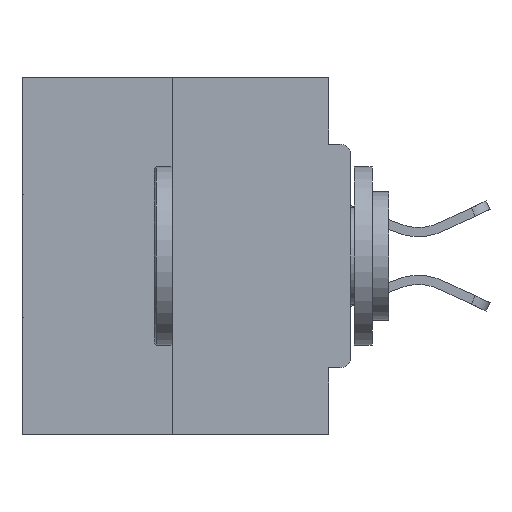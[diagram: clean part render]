
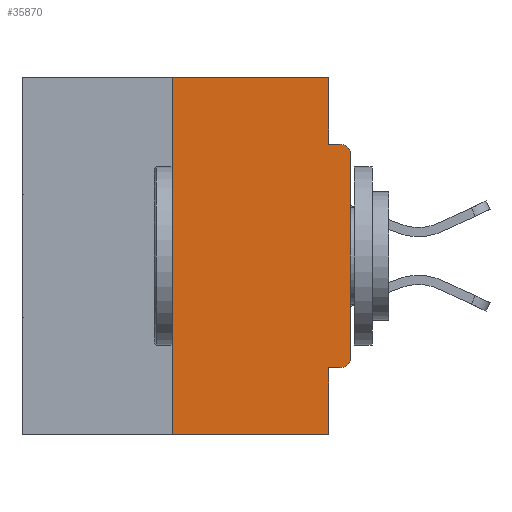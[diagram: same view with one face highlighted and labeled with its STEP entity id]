
A CAD part, left-side view. The second image highlights one B-rep face of the part: STEP entity #35870.
In plain terms, the highlighted planar face has unit normal (-1, 0, 0).
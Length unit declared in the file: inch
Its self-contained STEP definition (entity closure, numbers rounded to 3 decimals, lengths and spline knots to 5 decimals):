
#482 = VECTOR ( 'NONE', #6806, 39.37008 ) ;
#489 = EDGE_CURVE ( 'NONE', #1452, #10768, #7346, .T. ) ;
#610 = CARTESIAN_POINT ( 'NONE',  ( 0., 0.46, 0. ) ) ;
#1418 = CIRCLE ( 'NONE', #18785, 0.015 ) ;
#1452 = VERTEX_POINT ( 'NONE', #18834 ) ;
#1830 = DIRECTION ( 'NONE',  ( 0., -1., 0. ) ) ;
#2419 = CARTESIAN_POINT ( 'NONE',  ( 0., 0.031, 0. ) ) ;
#2492 = DIRECTION ( 'NONE',  ( 0., 0., -1. ) ) ;
#2782 = LINE ( 'NONE', #28223, #5684 ) ;
#2918 = VECTOR ( 'NONE', #22101, 39.37008 ) ;
#3023 = CARTESIAN_POINT ( 'NONE',  ( 0., 0.031, -0.5 ) ) ;
#3658 = EDGE_LOOP ( 'NONE', ( #23017, #25020, #5310, #17488, #17247, #20203, #36136, #10090, #22622, #37999 ) ) ;
#3687 = LINE ( 'NONE', #31050, #36047 ) ;
#4527 = LINE ( 'NONE', #3023, #8351 ) ;
#5092 = CARTESIAN_POINT ( 'NONE',  ( 0., 0.015, -0.3915 ) ) ;
#5310 = ORIENTED_EDGE ( 'NONE', *, *, #18344, .T. ) ;
#5544 = VERTEX_POINT ( 'NONE', #32115 ) ;
#5684 = VECTOR ( 'NONE', #31275, 39.37008 ) ;
#6282 = DIRECTION ( 'NONE',  ( 1., 0., 0. ) ) ;
#6806 = DIRECTION ( 'NONE',  ( 0., 0., 1. ) ) ;
#6832 = DIRECTION ( 'NONE',  ( 0., -1., 0. ) ) ;
#7287 = EDGE_CURVE ( 'NONE', #21469, #35300, #1418, .T. ) ;
#7346 = LINE ( 'NONE', #32718, #31035 ) ;
#7700 = LINE ( 'NONE', #34880, #482 ) ;
#7784 = LINE ( 'NONE', #2419, #22694 ) ;
#8351 = VECTOR ( 'NONE', #2492, 39.37008 ) ;
#9237 = VERTEX_POINT ( 'NONE', #31404 ) ;
#9278 = CARTESIAN_POINT ( 'NONE',  ( 0., 0., -0.4065 ) ) ;
#9405 = FACE_OUTER_BOUND ( 'NONE', #3658, .T. ) ;
#9901 = EDGE_CURVE ( 'NONE', #18406, #30310, #11078, .T. ) ;
#10090 = ORIENTED_EDGE ( 'NONE', *, *, #38746, .T. ) ;
#10210 = LINE ( 'NONE', #9278, #2918 ) ;
#10768 = VERTEX_POINT ( 'NONE', #24532 ) ;
#11078 = LINE ( 'NONE', #610, #33749 ) ;
#11183 = DIRECTION ( 'NONE',  ( 0., 0., -1. ) ) ;
#15640 = DIRECTION ( 'NONE',  ( 0., 0., -1. ) ) ;
#16112 = EDGE_CURVE ( 'NONE', #21469, #9237, #10210, .T. ) ;
#17247 = ORIENTED_EDGE ( 'NONE', *, *, #16112, .F. ) ;
#17488 = ORIENTED_EDGE ( 'NONE', *, *, #20269, .F. ) ;
#18344 = EDGE_CURVE ( 'NONE', #21398, #5544, #2782, .T. ) ;
#18406 = VERTEX_POINT ( 'NONE', #30561 ) ;
#18758 = PLANE ( 'NONE',  #30867 ) ;
#18785 = AXIS2_PLACEMENT_3D ( 'NONE', #5092, #36119, #11183 ) ;
#18821 = EDGE_CURVE ( 'NONE', #21398, #18406, #3687, .T. ) ;
#18834 = CARTESIAN_POINT ( 'NONE',  ( 0., 0.031, -0.0935 ) ) ;
#20203 = ORIENTED_EDGE ( 'NONE', *, *, #7287, .T. ) ;
#20269 = EDGE_CURVE ( 'NONE', #9237, #5544, #4527, .T. ) ;
#20296 = CARTESIAN_POINT ( 'NONE',  ( 0., 0., -0.1085 ) ) ;
#21398 = VERTEX_POINT ( 'NONE', #21840 ) ;
#21469 = VERTEX_POINT ( 'NONE', #26148 ) ;
#21644 = CARTESIAN_POINT ( 'NONE',  ( 0., 0.031, 0. ) ) ;
#21840 = CARTESIAN_POINT ( 'NONE',  ( 0., 0.25, -0.5 ) ) ;
#21857 = EDGE_CURVE ( 'NONE', #30310, #1452, #7784, .T. ) ;
#21949 = DIRECTION ( 'NONE',  ( 0., 0., -1. ) ) ;
#22101 = DIRECTION ( 'NONE',  ( 0., 1., 0. ) ) ;
#22309 = VERTEX_POINT ( 'NONE', #20296 ) ;
#22622 = ORIENTED_EDGE ( 'NONE', *, *, #489, .F. ) ;
#22694 = VECTOR ( 'NONE', #24458, 39.37008 ) ;
#22812 = DIRECTION ( 'NONE',  ( 0., 0., 1. ) ) ;
#23017 = ORIENTED_EDGE ( 'NONE', *, *, #9901, .F. ) ;
#23044 = EDGE_CURVE ( 'NONE', #35300, #22309, #7700, .T. ) ;
#24458 = DIRECTION ( 'NONE',  ( 0., 0., -1. ) ) ;
#24532 = CARTESIAN_POINT ( 'NONE',  ( 0., 0.015, -0.0935 ) ) ;
#24546 = DIRECTION ( 'NONE',  ( -1., 0., 0. ) ) ;
#24798 = CARTESIAN_POINT ( 'NONE',  ( 0., 0.46, 0. ) ) ;
#25020 = ORIENTED_EDGE ( 'NONE', *, *, #18821, .F. ) ;
#26148 = CARTESIAN_POINT ( 'NONE',  ( 0., 0.015, -0.4065 ) ) ;
#27881 = AXIS2_PLACEMENT_3D ( 'NONE', #33362, #24546, #15640 ) ;
#28223 = CARTESIAN_POINT ( 'NONE',  ( 0., 0.46, -0.5 ) ) ;
#30310 = VERTEX_POINT ( 'NONE', #21644 ) ;
#30561 = CARTESIAN_POINT ( 'NONE',  ( 0., 0.25, 0. ) ) ;
#30867 = AXIS2_PLACEMENT_3D ( 'NONE', #24798, #6282, #21949 ) ;
#31035 = VECTOR ( 'NONE', #1830, 39.37008 ) ;
#31050 = CARTESIAN_POINT ( 'NONE',  ( 0., 0.25, 0. ) ) ;
#31275 = DIRECTION ( 'NONE',  ( 0., -1., 0. ) ) ;
#31404 = CARTESIAN_POINT ( 'NONE',  ( 0., 0.031, -0.4065 ) ) ;
#32115 = CARTESIAN_POINT ( 'NONE',  ( 0., 0.031, -0.5 ) ) ;
#32648 = CARTESIAN_POINT ( 'NONE',  ( 0., 0., -0.3915 ) ) ;
#32718 = CARTESIAN_POINT ( 'NONE',  ( 0., 0., -0.0935 ) ) ;
#33362 = CARTESIAN_POINT ( 'NONE',  ( 0., 0.015, -0.1085 ) ) ;
#33749 = VECTOR ( 'NONE', #6832, 39.37008 ) ;
#34880 = CARTESIAN_POINT ( 'NONE',  ( 0., 0., 0. ) ) ;
#35300 = VERTEX_POINT ( 'NONE', #32648 ) ;
#35870 = ADVANCED_FACE ( 'NONE', ( #9405 ), #18758, .F. ) ;
#36047 = VECTOR ( 'NONE', #22812, 39.37008 ) ;
#36119 = DIRECTION ( 'NONE',  ( -1., 0., 0. ) ) ;
#36136 = ORIENTED_EDGE ( 'NONE', *, *, #23044, .T. ) ;
#37999 = ORIENTED_EDGE ( 'NONE', *, *, #21857, .F. ) ;
#38668 = CIRCLE ( 'NONE', #27881, 0.015 ) ;
#38746 = EDGE_CURVE ( 'NONE', #22309, #10768, #38668, .T. ) ;
